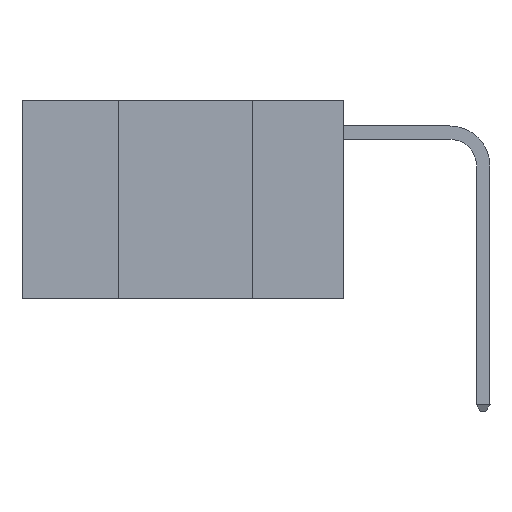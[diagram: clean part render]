
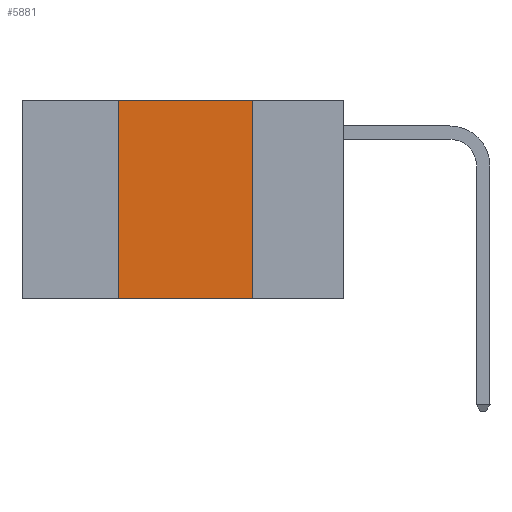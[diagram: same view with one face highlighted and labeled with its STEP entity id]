
A CAD part, left-side view. The second image highlights one B-rep face of the part: STEP entity #5881.
In plain terms, the highlighted planar face has unit normal (-1, 0, 0).
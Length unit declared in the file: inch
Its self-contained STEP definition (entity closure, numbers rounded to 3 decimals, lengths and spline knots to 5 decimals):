
#788 = VERTEX_POINT ( 'NONE', #5968 ) ;
#790 = VECTOR ( 'NONE', #7112, 39.37008 ) ;
#1502 = CARTESIAN_POINT ( 'NONE',  ( 0., 0.17, 0. ) ) ;
#2387 = VERTEX_POINT ( 'NONE', #26081 ) ;
#2549 = ORIENTED_EDGE ( 'NONE', *, *, #8555, .F. ) ;
#4076 = VECTOR ( 'NONE', #26200, 39.37008 ) ;
#4542 = CARTESIAN_POINT ( 'NONE',  ( 0., 0.42, 0. ) ) ;
#5013 = ORIENTED_EDGE ( 'NONE', *, *, #21812, .F. ) ;
#5256 = VERTEX_POINT ( 'NONE', #25534 ) ;
#5881 = ADVANCED_FACE ( 'NONE', ( #26040 ), #11443, .F. ) ;
#5968 = CARTESIAN_POINT ( 'NONE',  ( 0., 0.42, -0.37 ) ) ;
#6275 = EDGE_LOOP ( 'NONE', ( #27096, #2549, #5013, #24925 ) ) ;
#6760 = DIRECTION ( 'NONE',  ( 0., 0., -1. ) ) ;
#7033 = DIRECTION ( 'NONE',  ( 1., 0., 0. ) ) ;
#7112 = DIRECTION ( 'NONE',  ( 0., -1., 0. ) ) ;
#7567 = CARTESIAN_POINT ( 'NONE',  ( 0., 0.17, 0. ) ) ;
#8555 = EDGE_CURVE ( 'NONE', #2387, #26538, #11110, .T. ) ;
#8620 = CARTESIAN_POINT ( 'NONE',  ( 0., 0.6, 0. ) ) ;
#9426 = VECTOR ( 'NONE', #19424, 39.37008 ) ;
#9606 = DIRECTION ( 'NONE',  ( 0., 0., -1. ) ) ;
#11110 = LINE ( 'NONE', #8620, #790 ) ;
#11443 = PLANE ( 'NONE',  #20554 ) ;
#12496 = VECTOR ( 'NONE', #9606, 39.37008 ) ;
#16021 = LINE ( 'NONE', #22216, #4076 ) ;
#17625 = LINE ( 'NONE', #1502, #12496 ) ;
#19424 = DIRECTION ( 'NONE',  ( 0., 0., 1. ) ) ;
#19456 = CARTESIAN_POINT ( 'NONE',  ( 0., 0.6, 0. ) ) ;
#19770 = EDGE_CURVE ( 'NONE', #788, #5256, #16021, .T. ) ;
#20554 = AXIS2_PLACEMENT_3D ( 'NONE', #19456, #7033, #6760 ) ;
#21619 = LINE ( 'NONE', #4542, #9426 ) ;
#21812 = EDGE_CURVE ( 'NONE', #788, #2387, #21619, .T. ) ;
#21919 = EDGE_CURVE ( 'NONE', #26538, #5256, #17625, .T. ) ;
#22216 = CARTESIAN_POINT ( 'NONE',  ( 0., 0.6, -0.37 ) ) ;
#24925 = ORIENTED_EDGE ( 'NONE', *, *, #19770, .T. ) ;
#25534 = CARTESIAN_POINT ( 'NONE',  ( 0., 0.17, -0.37 ) ) ;
#26040 = FACE_OUTER_BOUND ( 'NONE', #6275, .T. ) ;
#26081 = CARTESIAN_POINT ( 'NONE',  ( 0., 0.42, 0. ) ) ;
#26200 = DIRECTION ( 'NONE',  ( 0., -1., 0. ) ) ;
#26538 = VERTEX_POINT ( 'NONE', #7567 ) ;
#27096 = ORIENTED_EDGE ( 'NONE', *, *, #21919, .F. ) ;
